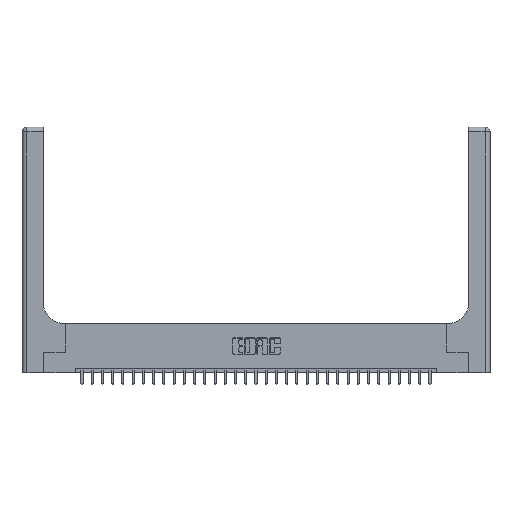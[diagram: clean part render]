
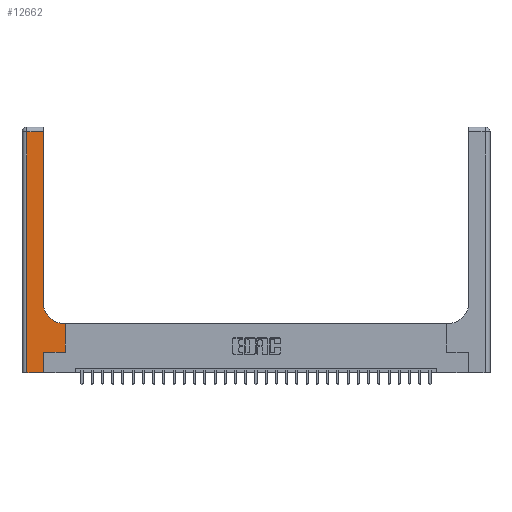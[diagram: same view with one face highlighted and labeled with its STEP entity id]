
A CAD part, top view. The second image highlights one B-rep face of the part: STEP entity #12662.
In plain terms, the highlighted planar face has unit normal (0, 0, 1).
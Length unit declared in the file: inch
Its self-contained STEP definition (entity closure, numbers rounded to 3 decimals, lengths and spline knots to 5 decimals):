
#344 = DIRECTION ( 'NONE',  ( 1., 0., 0. ) ) ;
#426 = ORIENTED_EDGE ( 'NONE', *, *, #4997, .T. ) ;
#483 = CARTESIAN_POINT ( 'NONE',  ( 0.51, 0.6, 0.37 ) ) ;
#560 = ORIENTED_EDGE ( 'NONE', *, *, #18347, .T. ) ;
#1205 = ORIENTED_EDGE ( 'NONE', *, *, #12133, .T. ) ;
#1564 = VECTOR ( 'NONE', #4830, 39.37008 ) ;
#1770 = EDGE_CURVE ( 'NONE', #24837, #5848, #19968, .T. ) ;
#1797 = CARTESIAN_POINT ( 'NONE',  ( 0.26, 0.85, 0.37 ) ) ;
#2194 = CARTESIAN_POINT ( 'NONE',  ( 0.06, 3., 0.37 ) ) ;
#2207 = CARTESIAN_POINT ( 'NONE',  ( 0.265, 0.25, 0.37 ) ) ;
#2627 = VECTOR ( 'NONE', #15078, 39.37008 ) ;
#2704 = ORIENTED_EDGE ( 'NONE', *, *, #20150, .T. ) ;
#4672 = DIRECTION ( 'NONE',  ( 0., -1., 0. ) ) ;
#4830 = DIRECTION ( 'NONE',  ( 1., 0., 0. ) ) ;
#4931 = CARTESIAN_POINT ( 'NONE',  ( 0.06, 0., 0.37 ) ) ;
#4997 = EDGE_CURVE ( 'NONE', #13938, #17240, #13493, .T. ) ;
#5848 = VERTEX_POINT ( 'NONE', #9165 ) ;
#5944 = CARTESIAN_POINT ( 'NONE',  ( 0.51, 0.85, 0.37 ) ) ;
#5967 = VERTEX_POINT ( 'NONE', #1797 ) ;
#7036 = VECTOR ( 'NONE', #12005, 39.37008 ) ;
#7194 = CARTESIAN_POINT ( 'NONE',  ( 0.528, 0.6, 0.37 ) ) ;
#7470 = PLANE ( 'NONE',  #20038 ) ;
#7789 = FACE_OUTER_BOUND ( 'NONE', #16658, .T. ) ;
#7799 = CARTESIAN_POINT ( 'NONE',  ( 0., 2.94, 0.37 ) ) ;
#7853 = VECTOR ( 'NONE', #13362, 39.37008 ) ;
#8163 = VERTEX_POINT ( 'NONE', #21227 ) ;
#8353 = ORIENTED_EDGE ( 'NONE', *, *, #17334, .T. ) ;
#9165 = CARTESIAN_POINT ( 'NONE',  ( 0.06, 2.94, 0.37 ) ) ;
#9549 = VECTOR ( 'NONE', #344, 39.37008 ) ;
#9578 = CARTESIAN_POINT ( 'NONE',  ( 0.26, 2.94, 0.37 ) ) ;
#9715 = ORIENTED_EDGE ( 'NONE', *, *, #20562, .T. ) ;
#9913 = LINE ( 'NONE', #14168, #7853 ) ;
#10519 = DIRECTION ( 'NONE',  ( 0., 0., -1. ) ) ;
#10622 = DIRECTION ( 'NONE',  ( -1., 0., 0. ) ) ;
#11222 = CIRCLE ( 'NONE', #16950, 0.25 ) ;
#11503 = EDGE_CURVE ( 'NONE', #24929, #8163, #27771, .T. ) ;
#12005 = DIRECTION ( 'NONE',  ( 0., 1., 0. ) ) ;
#12133 = EDGE_CURVE ( 'NONE', #5848, #13938, #22823, .T. ) ;
#12216 = ORIENTED_EDGE ( 'NONE', *, *, #20227, .T. ) ;
#12662 = ADVANCED_FACE ( 'NONE', ( #7789 ), #7470, .F. ) ;
#12686 = CARTESIAN_POINT ( 'NONE',  ( 0.265, 0., 0.37 ) ) ;
#13362 = DIRECTION ( 'NONE',  ( 0., 1., 0. ) ) ;
#13493 = LINE ( 'NONE', #15851, #1564 ) ;
#13827 = LINE ( 'NONE', #19940, #19026 ) ;
#13938 = VERTEX_POINT ( 'NONE', #4931 ) ;
#14151 = DIRECTION ( 'NONE',  ( -1., 0., 0. ) ) ;
#14168 = CARTESIAN_POINT ( 'NONE',  ( 0.528, 0.25, 0.37 ) ) ;
#14537 = VERTEX_POINT ( 'NONE', #483 ) ;
#15078 = DIRECTION ( 'NONE',  ( 0., 1., 0. ) ) ;
#15791 = LINE ( 'NONE', #25385, #7036 ) ;
#15851 = CARTESIAN_POINT ( 'NONE',  ( 0., 0., 0.37 ) ) ;
#16200 = VECTOR ( 'NONE', #4672, 39.37008 ) ;
#16658 = EDGE_LOOP ( 'NONE', ( #8353, #26351, #1205, #426, #2704, #24876, #9715, #560, #12216 ) ) ;
#16950 = AXIS2_PLACEMENT_3D ( 'NONE', #5944, #10519, #26296 ) ;
#17240 = VERTEX_POINT ( 'NONE', #12686 ) ;
#17334 = EDGE_CURVE ( 'NONE', #5967, #24837, #17354, .T. ) ;
#17354 = LINE ( 'NONE', #23715, #2627 ) ;
#18347 = EDGE_CURVE ( 'NONE', #22443, #14537, #13827, .T. ) ;
#19026 = VECTOR ( 'NONE', #10622, 39.37008 ) ;
#19940 = CARTESIAN_POINT ( 'NONE',  ( 0.26, 0.6, 0.37 ) ) ;
#19968 = LINE ( 'NONE', #7799, #28049 ) ;
#20038 = AXIS2_PLACEMENT_3D ( 'NONE', #23278, #23189, #14151 ) ;
#20150 = EDGE_CURVE ( 'NONE', #17240, #24929, #15791, .T. ) ;
#20227 = EDGE_CURVE ( 'NONE', #14537, #5967, #11222, .T. ) ;
#20562 = EDGE_CURVE ( 'NONE', #8163, #22443, #9913, .T. ) ;
#21227 = CARTESIAN_POINT ( 'NONE',  ( 0.528, 0.25, 0.37 ) ) ;
#22443 = VERTEX_POINT ( 'NONE', #7194 ) ;
#22823 = LINE ( 'NONE', #2194, #16200 ) ;
#23124 = DIRECTION ( 'NONE',  ( -1., 0., 0. ) ) ;
#23189 = DIRECTION ( 'NONE',  ( 0., 0., -1. ) ) ;
#23278 = CARTESIAN_POINT ( 'NONE',  ( 0., 3., 0.37 ) ) ;
#23715 = CARTESIAN_POINT ( 'NONE',  ( 0.26, 3., 0.37 ) ) ;
#24837 = VERTEX_POINT ( 'NONE', #9578 ) ;
#24876 = ORIENTED_EDGE ( 'NONE', *, *, #11503, .T. ) ;
#24929 = VERTEX_POINT ( 'NONE', #25011 ) ;
#25011 = CARTESIAN_POINT ( 'NONE',  ( 0.265, 0.25, 0.37 ) ) ;
#25385 = CARTESIAN_POINT ( 'NONE',  ( 0.265, 0., 0.37 ) ) ;
#26296 = DIRECTION ( 'NONE',  ( 1., 0., 0. ) ) ;
#26351 = ORIENTED_EDGE ( 'NONE', *, *, #1770, .T. ) ;
#27771 = LINE ( 'NONE', #2207, #9549 ) ;
#28049 = VECTOR ( 'NONE', #23124, 39.37008 ) ;
